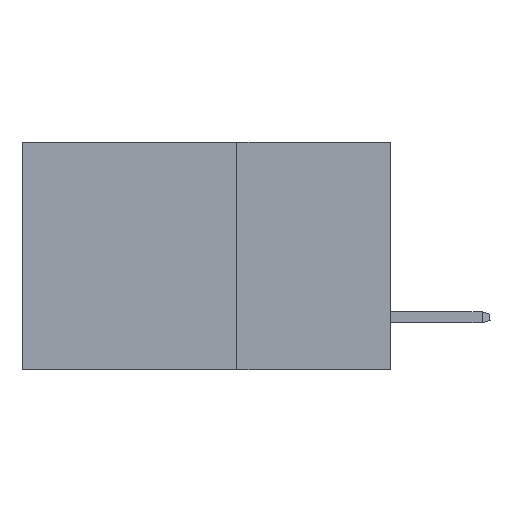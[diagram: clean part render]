
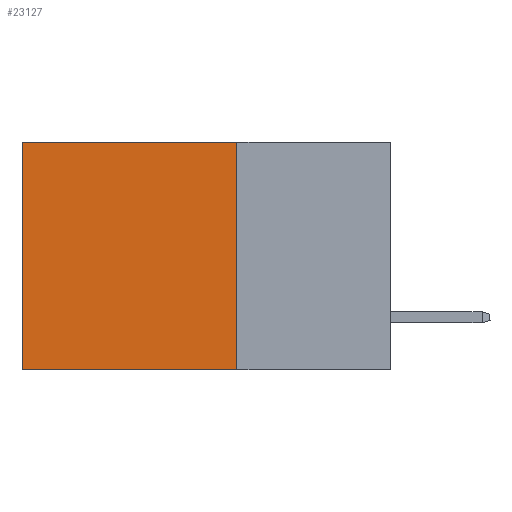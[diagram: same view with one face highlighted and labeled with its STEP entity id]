
A CAD part, left-side view. The second image highlights one B-rep face of the part: STEP entity #23127.
In plain terms, the highlighted planar face has unit normal (-1, 0, 0).
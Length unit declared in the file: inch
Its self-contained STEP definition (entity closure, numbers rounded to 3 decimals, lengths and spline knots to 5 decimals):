
#828 = CARTESIAN_POINT ( 'NONE',  ( 0.2875, 0.25, 0. ) ) ;
#1279 = ORIENTED_EDGE ( 'NONE', *, *, #3813, .F. ) ;
#2260 = LINE ( 'NONE', #25199, #25487 ) ;
#3803 = CARTESIAN_POINT ( 'NONE',  ( 0.2875, 0.25, 0. ) ) ;
#3813 = EDGE_CURVE ( 'NONE', #7602, #12193, #23491, .T. ) ;
#5066 = ORIENTED_EDGE ( 'NONE', *, *, #36760, .T. ) ;
#5264 = FACE_OUTER_BOUND ( 'NONE', #16051, .T. ) ;
#7602 = VERTEX_POINT ( 'NONE', #3803 ) ;
#8230 = EDGE_CURVE ( 'NONE', #7602, #25203, #33771, .T. ) ;
#8245 = EDGE_CURVE ( 'NONE', #12193, #18222, #9839, .T. ) ;
#8379 = VECTOR ( 'NONE', #38553, 39.37008 ) ;
#9839 = LINE ( 'NONE', #13097, #32845 ) ;
#12193 = VERTEX_POINT ( 'NONE', #28689 ) ;
#13097 = CARTESIAN_POINT ( 'NONE',  ( 0.2875, 0.25, -0.37 ) ) ;
#15951 = DIRECTION ( 'NONE',  ( 0., 0., -1. ) ) ;
#16051 = EDGE_LOOP ( 'NONE', ( #5066, #20841, #1279, #22898 ) ) ;
#18222 = VERTEX_POINT ( 'NONE', #29613 ) ;
#19579 = DIRECTION ( 'NONE',  ( 0., 0., -1. ) ) ;
#19770 = VECTOR ( 'NONE', #22062, 39.37008 ) ;
#19970 = CARTESIAN_POINT ( 'NONE',  ( 0.2875, 0.6, 0. ) ) ;
#20665 = CARTESIAN_POINT ( 'NONE',  ( 0.2875, 0.25, 0. ) ) ;
#20841 = ORIENTED_EDGE ( 'NONE', *, *, #8245, .F. ) ;
#22062 = DIRECTION ( 'NONE',  ( 0., 1., 0. ) ) ;
#22898 = ORIENTED_EDGE ( 'NONE', *, *, #8230, .T. ) ;
#23127 = ADVANCED_FACE ( 'NONE', ( #5264 ), #34475, .F. ) ;
#23491 = LINE ( 'NONE', #20665, #8379 ) ;
#25199 = CARTESIAN_POINT ( 'NONE',  ( 0.2875, 0.6, 0. ) ) ;
#25203 = VERTEX_POINT ( 'NONE', #19970 ) ;
#25487 = VECTOR ( 'NONE', #15951, 39.37008 ) ;
#28505 = CARTESIAN_POINT ( 'NONE',  ( 0.2875, 0.25, 0. ) ) ;
#28689 = CARTESIAN_POINT ( 'NONE',  ( 0.2875, 0.25, -0.37 ) ) ;
#29012 = AXIS2_PLACEMENT_3D ( 'NONE', #28505, #37500, #19579 ) ;
#29613 = CARTESIAN_POINT ( 'NONE',  ( 0.2875, 0.6, -0.37 ) ) ;
#31076 = DIRECTION ( 'NONE',  ( 0., 1., 0. ) ) ;
#32845 = VECTOR ( 'NONE', #31076, 39.37008 ) ;
#33771 = LINE ( 'NONE', #828, #19770 ) ;
#34475 = PLANE ( 'NONE',  #29012 ) ;
#36760 = EDGE_CURVE ( 'NONE', #25203, #18222, #2260, .T. ) ;
#37500 = DIRECTION ( 'NONE',  ( 1., 0., 0. ) ) ;
#38553 = DIRECTION ( 'NONE',  ( 0., 0., -1. ) ) ;
